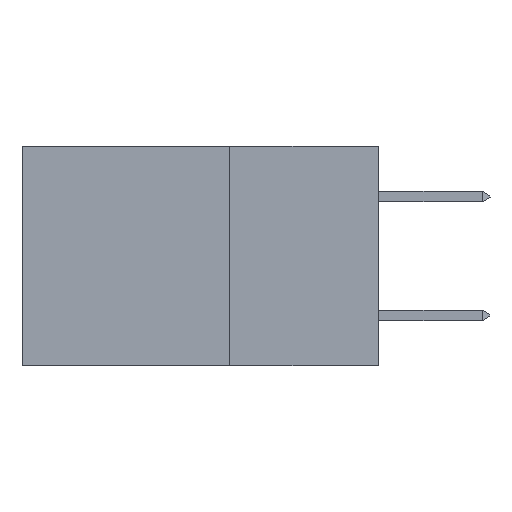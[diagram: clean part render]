
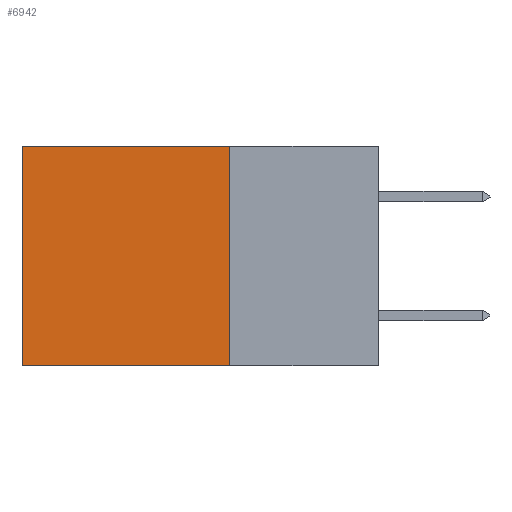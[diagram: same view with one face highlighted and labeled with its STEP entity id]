
A CAD part, left-side view. The second image highlights one B-rep face of the part: STEP entity #6942.
In plain terms, the highlighted planar face has unit normal (-1, 0, 0).
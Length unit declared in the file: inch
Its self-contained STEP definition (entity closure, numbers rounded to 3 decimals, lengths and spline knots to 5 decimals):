
#944 = ORIENTED_EDGE ( 'NONE', *, *, #4765, .F. ) ;
#2251 = ORIENTED_EDGE ( 'NONE', *, *, #11954, .T. ) ;
#3025 = CARTESIAN_POINT ( 'NONE',  ( 0.298, 0.6, 0. ) ) ;
#3092 = DIRECTION ( 'NONE',  ( 0., 0., -1. ) ) ;
#4402 = ORIENTED_EDGE ( 'NONE', *, *, #13706, .T. ) ;
#4582 = CARTESIAN_POINT ( 'NONE',  ( 0.298, 0.25, -0.37 ) ) ;
#4765 = EDGE_CURVE ( 'NONE', #27831, #10821, #20299, .T. ) ;
#6942 = ADVANCED_FACE ( 'NONE', ( #8822 ), #8065, .F. ) ;
#6953 = VECTOR ( 'NONE', #14216, 39.37008 ) ;
#7207 = EDGE_CURVE ( 'NONE', #17399, #27831, #7997, .T. ) ;
#7994 = CARTESIAN_POINT ( 'NONE',  ( 0.298, 0.25, 0. ) ) ;
#7997 = LINE ( 'NONE', #29685, #26606 ) ;
#8065 = PLANE ( 'NONE',  #21708 ) ;
#8822 = FACE_OUTER_BOUND ( 'NONE', #12879, .T. ) ;
#9993 = VECTOR ( 'NONE', #20290, 39.37008 ) ;
#10759 = ORIENTED_EDGE ( 'NONE', *, *, #7207, .F. ) ;
#10821 = VERTEX_POINT ( 'NONE', #27665 ) ;
#11954 = EDGE_CURVE ( 'NONE', #23216, #10821, #22775, .T. ) ;
#12879 = EDGE_LOOP ( 'NONE', ( #2251, #944, #10759, #4402 ) ) ;
#13706 = EDGE_CURVE ( 'NONE', #17399, #23216, #19313, .T. ) ;
#14216 = DIRECTION ( 'NONE',  ( 0., 1., 0. ) ) ;
#17399 = VERTEX_POINT ( 'NONE', #7994 ) ;
#17996 = CARTESIAN_POINT ( 'NONE',  ( 0.298, 0.25, 0. ) ) ;
#18237 = DIRECTION ( 'NONE',  ( 0., 1., 0. ) ) ;
#18758 = VECTOR ( 'NONE', #18237, 39.37008 ) ;
#19313 = LINE ( 'NONE', #31425, #6953 ) ;
#19893 = DIRECTION ( 'NONE',  ( 0., 0., -1. ) ) ;
#20290 = DIRECTION ( 'NONE',  ( 0., 0., -1. ) ) ;
#20299 = LINE ( 'NONE', #23905, #18758 ) ;
#21708 = AXIS2_PLACEMENT_3D ( 'NONE', #17996, #25170, #3092 ) ;
#22775 = LINE ( 'NONE', #3025, #9993 ) ;
#23216 = VERTEX_POINT ( 'NONE', #28661 ) ;
#23905 = CARTESIAN_POINT ( 'NONE',  ( 0.298, 0.25, -0.37 ) ) ;
#25170 = DIRECTION ( 'NONE',  ( 1., 0., 0. ) ) ;
#26606 = VECTOR ( 'NONE', #19893, 39.37008 ) ;
#27665 = CARTESIAN_POINT ( 'NONE',  ( 0.298, 0.6, -0.37 ) ) ;
#27831 = VERTEX_POINT ( 'NONE', #4582 ) ;
#28661 = CARTESIAN_POINT ( 'NONE',  ( 0.298, 0.6, 0. ) ) ;
#29685 = CARTESIAN_POINT ( 'NONE',  ( 0.298, 0.25, 0. ) ) ;
#31425 = CARTESIAN_POINT ( 'NONE',  ( 0.298, 0.25, 0. ) ) ;
